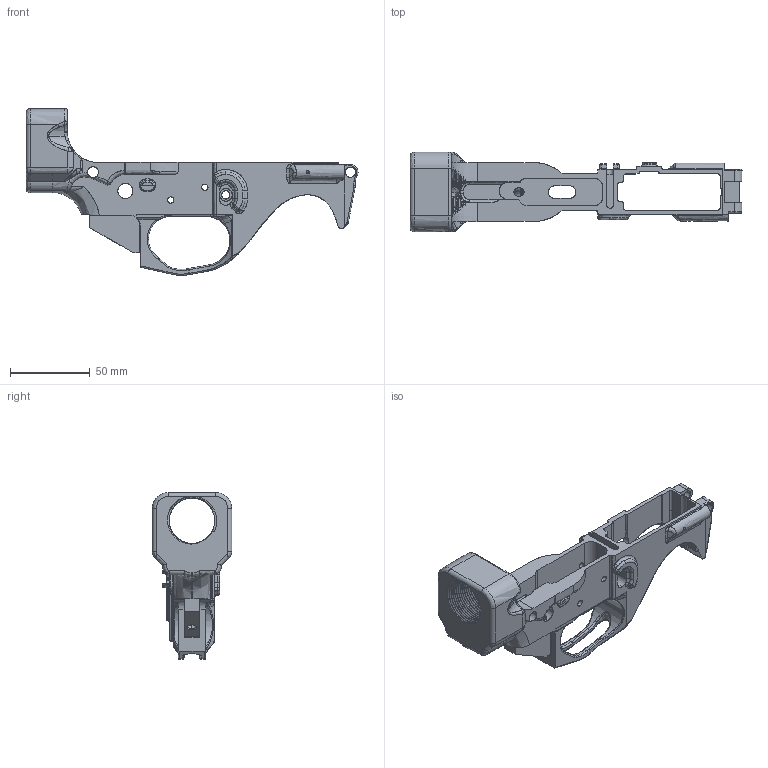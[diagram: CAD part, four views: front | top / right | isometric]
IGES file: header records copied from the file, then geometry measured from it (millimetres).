
Start section: SolidWorks IGES file using analytic representation for surfaces
Global section: file name: Hermes_Zero_V2.IGS; native system: SolidWorks 2015; preprocessor: SolidWorks 2015; author: WarFairy; date: 150521.113114; units: millimetre
Bounding box: 208.83 x 50 x 104.96 mm (x, y, z)
Surface area: 53704 mm2 (no closed solid volume)
Topology: 0 solids, 0 shells, 879 faces, 10428 edges, 10400 vertices
Faces by surface type: bspline 497, revolution 382
